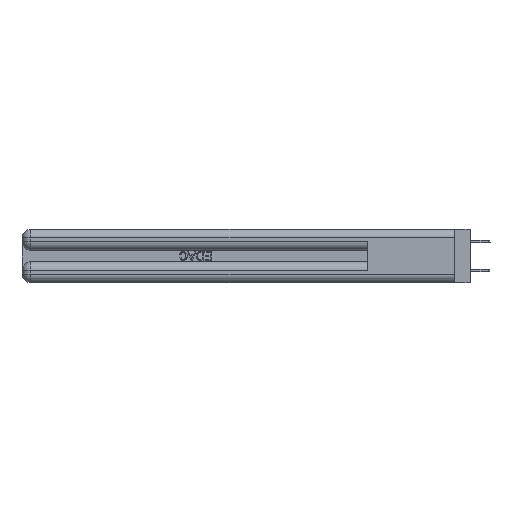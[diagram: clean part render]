
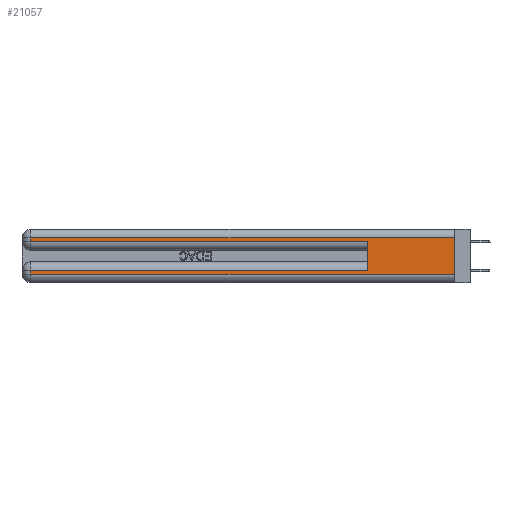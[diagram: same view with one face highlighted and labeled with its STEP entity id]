
A CAD part, left-side view. The second image highlights one B-rep face of the part: STEP entity #21057.
In plain terms, the highlighted planar face has unit normal (-1, 0, 0).
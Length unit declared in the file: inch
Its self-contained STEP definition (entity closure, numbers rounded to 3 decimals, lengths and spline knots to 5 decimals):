
#25 = CARTESIAN_POINT ( 'NONE',  ( 0., 0.6, 0.085 ) ) ;
#968 = ORIENTED_EDGE ( 'NONE', *, *, #8066, .T. ) ;
#2213 = CARTESIAN_POINT ( 'NONE',  ( 0., 0., 0.31 ) ) ;
#2746 = CARTESIAN_POINT ( 'NONE',  ( 0., 2.94, 0.37 ) ) ;
#2845 = VECTOR ( 'NONE', #32432, 39.37008 ) ;
#4326 = EDGE_CURVE ( 'NONE', #7016, #33720, #32681, .T. ) ;
#5430 = ORIENTED_EDGE ( 'NONE', *, *, #35147, .F. ) ;
#5868 = CARTESIAN_POINT ( 'NONE',  ( 0., 2.94, 0.37 ) ) ;
#6336 = DIRECTION ( 'NONE',  ( 0., 1., 0. ) ) ;
#7016 = VERTEX_POINT ( 'NONE', #25 ) ;
#8066 = EDGE_CURVE ( 'NONE', #25885, #14429, #38157, .T. ) ;
#8279 = ORIENTED_EDGE ( 'NONE', *, *, #4326, .T. ) ;
#8797 = ORIENTED_EDGE ( 'NONE', *, *, #46485, .T. ) ;
#10375 = DIRECTION ( 'NONE',  ( 1., 0., 0. ) ) ;
#10540 = VECTOR ( 'NONE', #17239, 39.37008 ) ;
#10635 = CARTESIAN_POINT ( 'NONE',  ( 0., 2.94, 0.285 ) ) ;
#14429 = VERTEX_POINT ( 'NONE', #44320 ) ;
#14777 = DIRECTION ( 'NONE',  ( 0., 0., -1. ) ) ;
#15455 = CARTESIAN_POINT ( 'NONE',  ( 0., 0., 0.06 ) ) ;
#16543 = EDGE_CURVE ( 'NONE', #35603, #28571, #23164, .T. ) ;
#16702 = EDGE_CURVE ( 'NONE', #26482, #38370, #21096, .T. ) ;
#17239 = DIRECTION ( 'NONE',  ( 0., -1., 0. ) ) ;
#18437 = DIRECTION ( 'NONE',  ( 0., 0., -1. ) ) ;
#19799 = VECTOR ( 'NONE', #18437, 39.37008 ) ;
#20312 = CARTESIAN_POINT ( 'NONE',  ( 0., 2.94, 0.06 ) ) ;
#21057 = ADVANCED_FACE ( 'NONE', ( #25790 ), #49659, .F. ) ;
#21096 = LINE ( 'NONE', #21599, #10540 ) ;
#21599 = CARTESIAN_POINT ( 'NONE',  ( 0., 0., 0.285 ) ) ;
#21753 = CARTESIAN_POINT ( 'NONE',  ( 0., 0., 0.37 ) ) ;
#23164 = LINE ( 'NONE', #15455, #40905 ) ;
#24940 = VECTOR ( 'NONE', #14777, 39.37008 ) ;
#25669 = ORIENTED_EDGE ( 'NONE', *, *, #49556, .F. ) ;
#25790 = FACE_OUTER_BOUND ( 'NONE', #42460, .T. ) ;
#25885 = VERTEX_POINT ( 'NONE', #36687 ) ;
#26482 = VERTEX_POINT ( 'NONE', #10635 ) ;
#26484 = ORIENTED_EDGE ( 'NONE', *, *, #16702, .T. ) ;
#27072 = VECTOR ( 'NONE', #39637, 39.37008 ) ;
#27313 = LINE ( 'NONE', #43232, #27072 ) ;
#28571 = VERTEX_POINT ( 'NONE', #34995 ) ;
#29663 = DIRECTION ( 'NONE',  ( 0., 0., -1. ) ) ;
#29922 = CARTESIAN_POINT ( 'NONE',  ( 0., 0., 0.37 ) ) ;
#32432 = DIRECTION ( 'NONE',  ( 0., 1., 0. ) ) ;
#32542 = AXIS2_PLACEMENT_3D ( 'NONE', #29922, #10375, #29663 ) ;
#32681 = LINE ( 'NONE', #36266, #2845 ) ;
#33530 = ORIENTED_EDGE ( 'NONE', *, *, #16543, .T. ) ;
#33720 = VERTEX_POINT ( 'NONE', #47320 ) ;
#34108 = DIRECTION ( 'NONE',  ( 0., 0., -1. ) ) ;
#34118 = LINE ( 'NONE', #5868, #19799 ) ;
#34240 = DIRECTION ( 'NONE',  ( 0., -1., 0. ) ) ;
#34995 = CARTESIAN_POINT ( 'NONE',  ( 0., 0., 0.06 ) ) ;
#35147 = EDGE_CURVE ( 'NONE', #7016, #38370, #27313, .T. ) ;
#35603 = VERTEX_POINT ( 'NONE', #20312 ) ;
#36266 = CARTESIAN_POINT ( 'NONE',  ( 0., 0., 0.085 ) ) ;
#36687 = CARTESIAN_POINT ( 'NONE',  ( 0., 0., 0.31 ) ) ;
#37042 = ORIENTED_EDGE ( 'NONE', *, *, #42528, .T. ) ;
#37182 = VECTOR ( 'NONE', #6336, 39.37008 ) ;
#38157 = LINE ( 'NONE', #2213, #37182 ) ;
#38370 = VERTEX_POINT ( 'NONE', #43562 ) ;
#38410 = LINE ( 'NONE', #21753, #24940 ) ;
#38442 = LINE ( 'NONE', #2746, #50364 ) ;
#39637 = DIRECTION ( 'NONE',  ( 0., 0., 1. ) ) ;
#40905 = VECTOR ( 'NONE', #34240, 39.37008 ) ;
#42460 = EDGE_LOOP ( 'NONE', ( #25669, #968, #8797, #26484, #5430, #8279, #37042, #33530 ) ) ;
#42528 = EDGE_CURVE ( 'NONE', #33720, #35603, #38442, .T. ) ;
#43232 = CARTESIAN_POINT ( 'NONE',  ( 0., 0.6, 0.145 ) ) ;
#43562 = CARTESIAN_POINT ( 'NONE',  ( 0., 0.6, 0.285 ) ) ;
#44320 = CARTESIAN_POINT ( 'NONE',  ( 0., 2.94, 0.31 ) ) ;
#46485 = EDGE_CURVE ( 'NONE', #14429, #26482, #34118, .T. ) ;
#47320 = CARTESIAN_POINT ( 'NONE',  ( 0., 2.94, 0.085 ) ) ;
#49556 = EDGE_CURVE ( 'NONE', #25885, #28571, #38410, .T. ) ;
#49659 = PLANE ( 'NONE',  #32542 ) ;
#50364 = VECTOR ( 'NONE', #34108, 39.37008 ) ;
